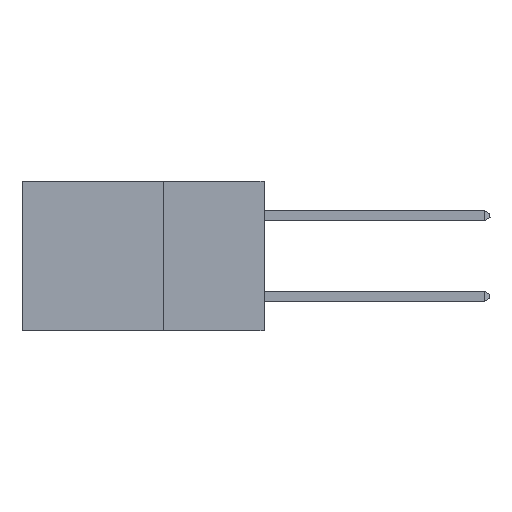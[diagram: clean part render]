
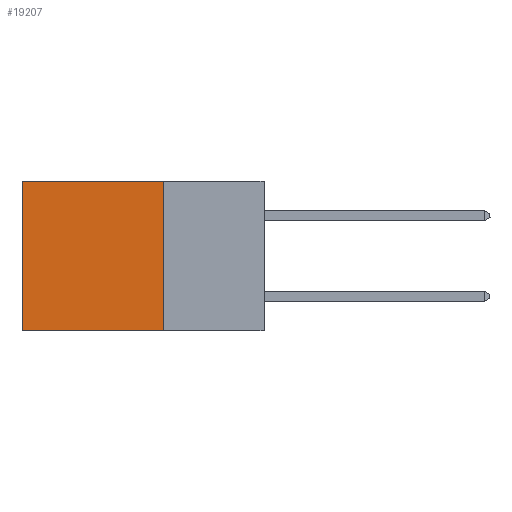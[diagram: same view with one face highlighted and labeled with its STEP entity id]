
A CAD part, left-side view. The second image highlights one B-rep face of the part: STEP entity #19207.
In plain terms, the highlighted planar face has unit normal (-1, 0, 0).
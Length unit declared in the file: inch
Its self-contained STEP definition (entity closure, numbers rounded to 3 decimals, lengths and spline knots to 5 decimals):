
#138 = CARTESIAN_POINT ( 'NONE',  ( 0.298, 0.25, -0.37 ) ) ;
#938 = CARTESIAN_POINT ( 'NONE',  ( 0.298, 0.25, -0.37 ) ) ;
#1210 = ORIENTED_EDGE ( 'NONE', *, *, #4525, .F. ) ;
#1871 = DIRECTION ( 'NONE',  ( 0., 0., -1. ) ) ;
#2855 = EDGE_CURVE ( 'NONE', #4748, #8078, #19119, .T. ) ;
#3790 = VECTOR ( 'NONE', #5923, 39.37008 ) ;
#3866 = EDGE_CURVE ( 'NONE', #17156, #13864, #10526, .T. ) ;
#4340 = CARTESIAN_POINT ( 'NONE',  ( 0.298, 0.25, 0. ) ) ;
#4525 = EDGE_CURVE ( 'NONE', #13864, #8078, #6198, .T. ) ;
#4540 = AXIS2_PLACEMENT_3D ( 'NONE', #9028, #18132, #14894 ) ;
#4748 = VERTEX_POINT ( 'NONE', #6462 ) ;
#4990 = CARTESIAN_POINT ( 'NONE',  ( 0.298, 0.6, 0. ) ) ;
#5370 = VECTOR ( 'NONE', #1871, 39.37008 ) ;
#5414 = EDGE_CURVE ( 'NONE', #17156, #4748, #6382, .T. ) ;
#5923 = DIRECTION ( 'NONE',  ( 0., 1., 0. ) ) ;
#6067 = DIRECTION ( 'NONE',  ( 0., 1., 0. ) ) ;
#6198 = LINE ( 'NONE', #138, #19489 ) ;
#6382 = LINE ( 'NONE', #4340, #3790 ) ;
#6445 = DIRECTION ( 'NONE',  ( 0., 0., -1. ) ) ;
#6462 = CARTESIAN_POINT ( 'NONE',  ( 0.298, 0.6, 0. ) ) ;
#7436 = PLANE ( 'NONE',  #4540 ) ;
#8025 = CARTESIAN_POINT ( 'NONE',  ( 0.298, 0.25, 0. ) ) ;
#8061 = ORIENTED_EDGE ( 'NONE', *, *, #2855, .T. ) ;
#8078 = VERTEX_POINT ( 'NONE', #17068 ) ;
#9028 = CARTESIAN_POINT ( 'NONE',  ( 0.298, 0.25, 0. ) ) ;
#9052 = ORIENTED_EDGE ( 'NONE', *, *, #3866, .F. ) ;
#10526 = LINE ( 'NONE', #8025, #15025 ) ;
#10667 = FACE_OUTER_BOUND ( 'NONE', #12871, .T. ) ;
#12871 = EDGE_LOOP ( 'NONE', ( #8061, #1210, #9052, #14912 ) ) ;
#13864 = VERTEX_POINT ( 'NONE', #938 ) ;
#14228 = CARTESIAN_POINT ( 'NONE',  ( 0.298, 0.25, 0. ) ) ;
#14894 = DIRECTION ( 'NONE',  ( 0., 0., -1. ) ) ;
#14912 = ORIENTED_EDGE ( 'NONE', *, *, #5414, .T. ) ;
#15025 = VECTOR ( 'NONE', #6445, 39.37008 ) ;
#17068 = CARTESIAN_POINT ( 'NONE',  ( 0.298, 0.6, -0.37 ) ) ;
#17156 = VERTEX_POINT ( 'NONE', #14228 ) ;
#18132 = DIRECTION ( 'NONE',  ( 1., 0., 0. ) ) ;
#19119 = LINE ( 'NONE', #4990, #5370 ) ;
#19207 = ADVANCED_FACE ( 'NONE', ( #10667 ), #7436, .F. ) ;
#19489 = VECTOR ( 'NONE', #6067, 39.37008 ) ;
